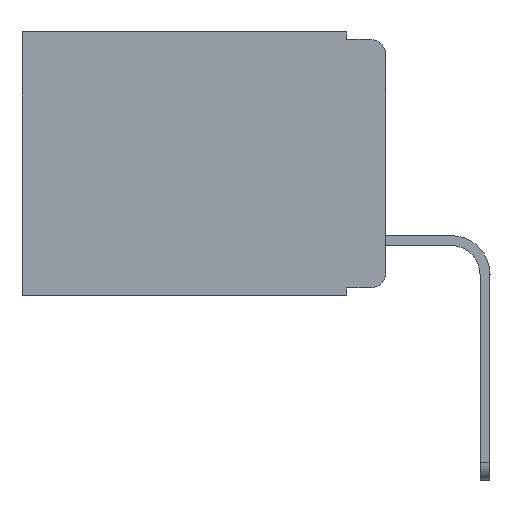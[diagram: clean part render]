
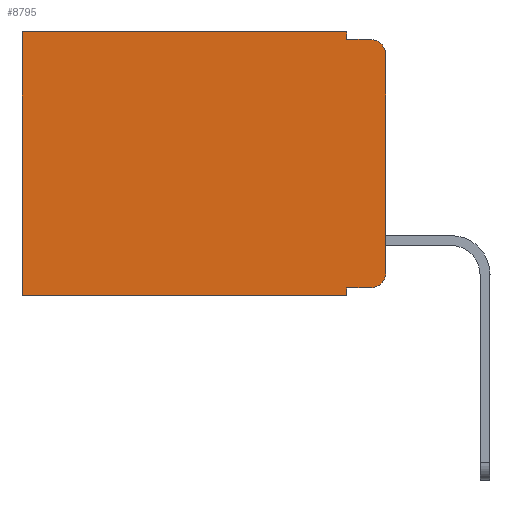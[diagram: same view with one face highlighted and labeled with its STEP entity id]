
A CAD part, left-side view. The second image highlights one B-rep face of the part: STEP entity #8795.
In plain terms, the highlighted planar face has unit normal (-1, 0, 0).
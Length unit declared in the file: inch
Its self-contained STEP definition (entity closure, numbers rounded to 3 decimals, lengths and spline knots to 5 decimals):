
#297 = CARTESIAN_POINT ( 'NONE',  ( 0.298, 0., -0.03 ) ) ;
#358 = DIRECTION ( 'NONE',  ( -1., 0., 0. ) ) ;
#559 = VERTEX_POINT ( 'NONE', #13181 ) ;
#672 = CARTESIAN_POINT ( 'NONE',  ( 0.298, 0.473, 0. ) ) ;
#773 = AXIS2_PLACEMENT_3D ( 'NONE', #11334, #358, #3585 ) ;
#1031 = EDGE_LOOP ( 'NONE', ( #8568, #4005, #14193, #13470, #7529, #3310, #10338, #6816, #9961, #3403 ) ) ;
#1056 = VECTOR ( 'NONE', #2987, 39.37008 ) ;
#1727 = DIRECTION ( 'NONE',  ( 0., 0., -1. ) ) ;
#1800 = VERTEX_POINT ( 'NONE', #8606 ) ;
#1851 = VECTOR ( 'NONE', #2246, 39.37008 ) ;
#2047 = EDGE_CURVE ( 'NONE', #13242, #5558, #12916, .T. ) ;
#2246 = DIRECTION ( 'NONE',  ( 0., -1., 0. ) ) ;
#2340 = DIRECTION ( 'NONE',  ( 0., 0., -1. ) ) ;
#2844 = CARTESIAN_POINT ( 'NONE',  ( 0.298, 0.02, -0.03 ) ) ;
#2935 = VECTOR ( 'NONE', #1727, 39.37008 ) ;
#2987 = DIRECTION ( 'NONE',  ( 0., 0., -1. ) ) ;
#3148 = CARTESIAN_POINT ( 'NONE',  ( 0.298, 0., 0. ) ) ;
#3201 = CARTESIAN_POINT ( 'NONE',  ( 0.298, 0.051, 0. ) ) ;
#3310 = ORIENTED_EDGE ( 'NONE', *, *, #6971, .T. ) ;
#3403 = ORIENTED_EDGE ( 'NONE', *, *, #10511, .T. ) ;
#3478 = CARTESIAN_POINT ( 'NONE',  ( 0.298, 0.02, -0.01 ) ) ;
#3585 = DIRECTION ( 'NONE',  ( 0., 0., -1. ) ) ;
#4005 = ORIENTED_EDGE ( 'NONE', *, *, #5265, .T. ) ;
#4010 = LINE ( 'NONE', #12610, #14028 ) ;
#4145 = DIRECTION ( 'NONE',  ( 0., 1., 0. ) ) ;
#5153 = DIRECTION ( 'NONE',  ( 0., 0., -1. ) ) ;
#5249 = DIRECTION ( 'NONE',  ( 0., 0., -1. ) ) ;
#5265 = EDGE_CURVE ( 'NONE', #6776, #5558, #8443, .T. ) ;
#5266 = CARTESIAN_POINT ( 'NONE',  ( 0.298, 0.051, -0.01 ) ) ;
#5281 = EDGE_CURVE ( 'NONE', #6776, #9518, #13861, .T. ) ;
#5558 = VERTEX_POINT ( 'NONE', #3478 ) ;
#5665 = EDGE_CURVE ( 'NONE', #6295, #1800, #4010, .T. ) ;
#5866 = DIRECTION ( 'NONE',  ( 0., -1., 0. ) ) ;
#5936 = VERTEX_POINT ( 'NONE', #672 ) ;
#6295 = VERTEX_POINT ( 'NONE', #8430 ) ;
#6373 = CIRCLE ( 'NONE', #773, 0.02 ) ;
#6446 = CARTESIAN_POINT ( 'NONE',  ( 0.298, 0., 0. ) ) ;
#6467 = DIRECTION ( 'NONE',  ( 0., 1., 0. ) ) ;
#6641 = VECTOR ( 'NONE', #2340, 39.37008 ) ;
#6776 = VERTEX_POINT ( 'NONE', #297 ) ;
#6816 = ORIENTED_EDGE ( 'NONE', *, *, #13008, .F. ) ;
#6971 = EDGE_CURVE ( 'NONE', #5936, #559, #13312, .T. ) ;
#7373 = CARTESIAN_POINT ( 'NONE',  ( 0.298, 0.473, 0. ) ) ;
#7500 = LINE ( 'NONE', #13089, #9951 ) ;
#7529 = ORIENTED_EDGE ( 'NONE', *, *, #10178, .T. ) ;
#7572 = CARTESIAN_POINT ( 'NONE',  ( 0.298, 0.051, 0. ) ) ;
#7682 = EDGE_CURVE ( 'NONE', #11838, #559, #7500, .T. ) ;
#7707 = VERTEX_POINT ( 'NONE', #3201 ) ;
#7954 = LINE ( 'NONE', #7572, #9169 ) ;
#8430 = CARTESIAN_POINT ( 'NONE',  ( 0.298, 0.051, -0.333 ) ) ;
#8443 = CIRCLE ( 'NONE', #12433, 0.02 ) ;
#8561 = PLANE ( 'NONE',  #14165 ) ;
#8568 = ORIENTED_EDGE ( 'NONE', *, *, #5281, .F. ) ;
#8606 = CARTESIAN_POINT ( 'NONE',  ( 0.298, 0.02, -0.333 ) ) ;
#8795 = ADVANCED_FACE ( 'NONE', ( #11312 ), #8561, .F. ) ;
#8981 = CARTESIAN_POINT ( 'NONE',  ( 0.298, 0.051, -0.01 ) ) ;
#9169 = VECTOR ( 'NONE', #9624, 39.37008 ) ;
#9361 = LINE ( 'NONE', #3148, #14432 ) ;
#9391 = CARTESIAN_POINT ( 'NONE',  ( 0.298, 0., 0. ) ) ;
#9518 = VERTEX_POINT ( 'NONE', #14110 ) ;
#9624 = DIRECTION ( 'NONE',  ( 0., 0., -1. ) ) ;
#9671 = DIRECTION ( 'NONE',  ( -1., 0., 0. ) ) ;
#9951 = VECTOR ( 'NONE', #4145, 39.37008 ) ;
#9961 = ORIENTED_EDGE ( 'NONE', *, *, #5665, .T. ) ;
#10175 = CARTESIAN_POINT ( 'NONE',  ( 0.298, 0.051, 0. ) ) ;
#10178 = EDGE_CURVE ( 'NONE', #7707, #5936, #9361, .T. ) ;
#10338 = ORIENTED_EDGE ( 'NONE', *, *, #7682, .F. ) ;
#10511 = EDGE_CURVE ( 'NONE', #1800, #9518, #6373, .T. ) ;
#10783 = EDGE_CURVE ( 'NONE', #7707, #13242, #7954, .T. ) ;
#11312 = FACE_OUTER_BOUND ( 'NONE', #1031, .T. ) ;
#11334 = CARTESIAN_POINT ( 'NONE',  ( 0.298, 0.02, -0.313 ) ) ;
#11691 = CARTESIAN_POINT ( 'NONE',  ( 0.298, 0.051, -0.343 ) ) ;
#11838 = VERTEX_POINT ( 'NONE', #11691 ) ;
#11926 = DIRECTION ( 'NONE',  ( 1., 0., 0. ) ) ;
#12062 = LINE ( 'NONE', #10175, #6641 ) ;
#12433 = AXIS2_PLACEMENT_3D ( 'NONE', #2844, #9671, #5153 ) ;
#12610 = CARTESIAN_POINT ( 'NONE',  ( 0.298, 0.051, -0.333 ) ) ;
#12916 = LINE ( 'NONE', #8981, #1851 ) ;
#13008 = EDGE_CURVE ( 'NONE', #6295, #11838, #12062, .T. ) ;
#13089 = CARTESIAN_POINT ( 'NONE',  ( 0.298, 0., -0.343 ) ) ;
#13181 = CARTESIAN_POINT ( 'NONE',  ( 0.298, 0.473, -0.343 ) ) ;
#13242 = VERTEX_POINT ( 'NONE', #5266 ) ;
#13312 = LINE ( 'NONE', #7373, #2935 ) ;
#13470 = ORIENTED_EDGE ( 'NONE', *, *, #10783, .F. ) ;
#13861 = LINE ( 'NONE', #9391, #1056 ) ;
#14028 = VECTOR ( 'NONE', #5866, 39.37008 ) ;
#14110 = CARTESIAN_POINT ( 'NONE',  ( 0.298, 0., -0.313 ) ) ;
#14165 = AXIS2_PLACEMENT_3D ( 'NONE', #6446, #11926, #5249 ) ;
#14193 = ORIENTED_EDGE ( 'NONE', *, *, #2047, .F. ) ;
#14432 = VECTOR ( 'NONE', #6467, 39.37008 ) ;
